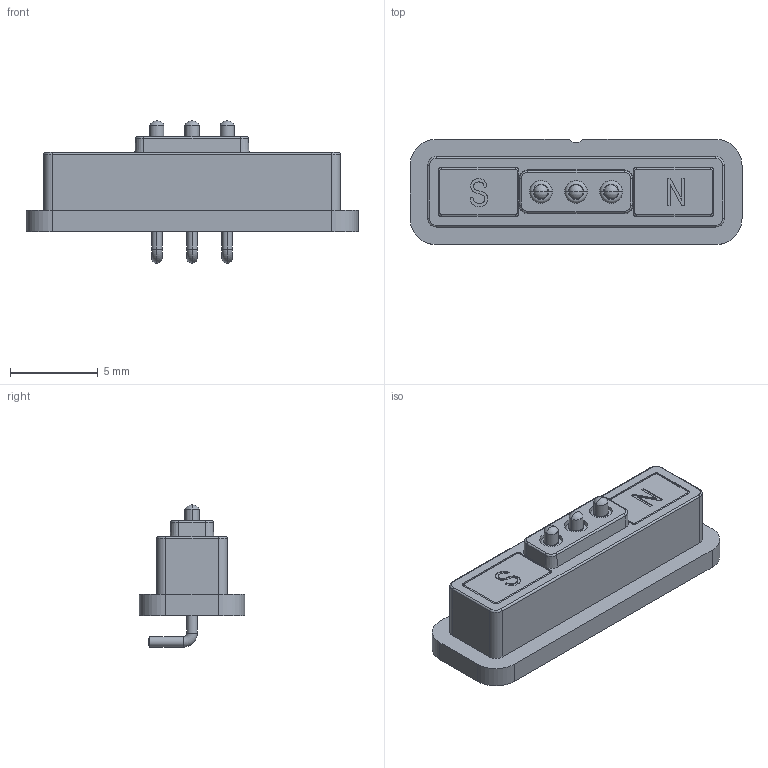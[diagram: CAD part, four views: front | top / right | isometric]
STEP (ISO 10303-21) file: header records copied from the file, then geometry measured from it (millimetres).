
FILE_DESCRIPTION (( 'STEP AP214' ), '1' );
FILE_NAME ('685F0321351120E.STEP', '2023-04-12T13:50:43', ( '' ), ( '' ), 'SwSTEP 2.0', 'SolidWorks 2020', '' );
FILE_SCHEMA (( 'AUTOMOTIVE_DESIGN' ));
Length unit declared in the file: millimetre
Products named in the file (1): 685F0321351120E
Bounding box: 18.9 x 6 x 8.1 mm (x, y, z)
Volume: 342.4 mm3; surface area: 626.6 mm2
Topology: 4 solids, 9 shells, 264 faces, 595 edges, 364 vertices
Faces by surface type: cylinder 105, plane 87, torus 36, cone 16, bspline 14, sphere 6
Entity records: 11018 total; most frequent: CARTESIAN_POINT 2054, DIRECTION 1338, ORIENTED_EDGE 1190, EDGE_CURVE 595, AXIS2_PLACEMENT_3D 520, VERTEX_POINT 364, VECTOR 298, LINE 298
